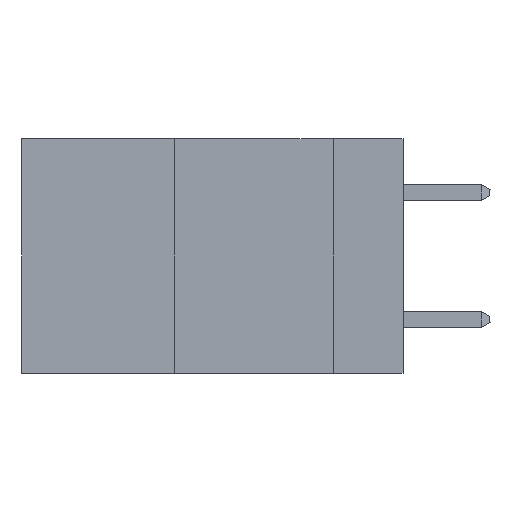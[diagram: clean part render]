
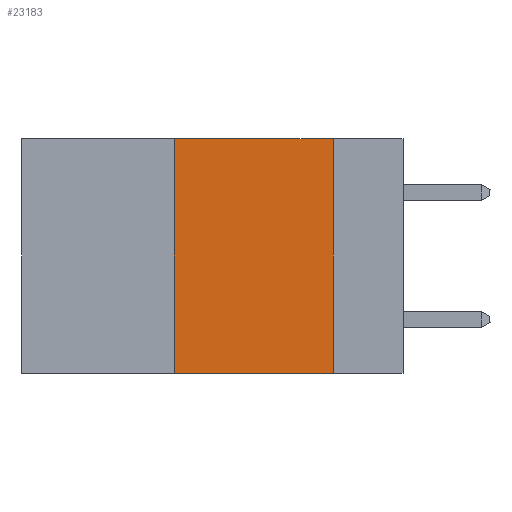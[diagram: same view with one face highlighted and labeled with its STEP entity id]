
A CAD part, left-side view. The second image highlights one B-rep face of the part: STEP entity #23183.
In plain terms, the highlighted planar face has unit normal (-1, 0, 0).
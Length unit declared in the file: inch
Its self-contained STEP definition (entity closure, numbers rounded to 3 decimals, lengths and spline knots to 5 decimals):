
#1402 = DIRECTION ( 'NONE',  ( 0., 0., -1. ) ) ;
#1811 = CARTESIAN_POINT ( 'NONE',  ( 0., 0.6, 0. ) ) ;
#2018 = EDGE_CURVE ( 'NONE', #37760, #12772, #20050, .T. ) ;
#2863 = EDGE_CURVE ( 'NONE', #10679, #37760, #13141, .T. ) ;
#3066 = VECTOR ( 'NONE', #6908, 39.37008 ) ;
#6908 = DIRECTION ( 'NONE',  ( 0., 0., 1. ) ) ;
#8728 = VECTOR ( 'NONE', #30118, 39.37008 ) ;
#8920 = EDGE_CURVE ( 'NONE', #46099, #10679, #19855, .T. ) ;
#9226 = CARTESIAN_POINT ( 'NONE',  ( 0., 0.36, -0.37 ) ) ;
#10679 = VERTEX_POINT ( 'NONE', #29574 ) ;
#11823 = AXIS2_PLACEMENT_3D ( 'NONE', #1811, #25742, #17429 ) ;
#12772 = VERTEX_POINT ( 'NONE', #44998 ) ;
#13032 = CARTESIAN_POINT ( 'NONE',  ( 0., 0.11, 0. ) ) ;
#13141 = LINE ( 'NONE', #18152, #8728 ) ;
#15585 = ORIENTED_EDGE ( 'NONE', *, *, #2018, .F. ) ;
#17429 = DIRECTION ( 'NONE',  ( 0., 0., -1. ) ) ;
#17936 = PLANE ( 'NONE',  #11823 ) ;
#18152 = CARTESIAN_POINT ( 'NONE',  ( 0., 0.6, 0. ) ) ;
#19242 = CARTESIAN_POINT ( 'NONE',  ( 0., 0.36, 0. ) ) ;
#19348 = EDGE_LOOP ( 'NONE', ( #15585, #40892, #36220, #49140 ) ) ;
#19855 = LINE ( 'NONE', #19242, #3066 ) ;
#20050 = LINE ( 'NONE', #25315, #39928 ) ;
#21603 = EDGE_CURVE ( 'NONE', #46099, #12772, #36631, .T. ) ;
#23014 = CARTESIAN_POINT ( 'NONE',  ( 0., 0.6, -0.37 ) ) ;
#23183 = ADVANCED_FACE ( 'NONE', ( #37629 ), #17936, .F. ) ;
#25315 = CARTESIAN_POINT ( 'NONE',  ( 0., 0.11, 0. ) ) ;
#25742 = DIRECTION ( 'NONE',  ( 1., 0., 0. ) ) ;
#29574 = CARTESIAN_POINT ( 'NONE',  ( 0., 0.36, 0. ) ) ;
#30118 = DIRECTION ( 'NONE',  ( 0., -1., 0. ) ) ;
#31193 = DIRECTION ( 'NONE',  ( 0., -1., 0. ) ) ;
#36220 = ORIENTED_EDGE ( 'NONE', *, *, #8920, .F. ) ;
#36631 = LINE ( 'NONE', #23014, #42222 ) ;
#37629 = FACE_OUTER_BOUND ( 'NONE', #19348, .T. ) ;
#37760 = VERTEX_POINT ( 'NONE', #13032 ) ;
#39928 = VECTOR ( 'NONE', #1402, 39.37008 ) ;
#40892 = ORIENTED_EDGE ( 'NONE', *, *, #2863, .F. ) ;
#42222 = VECTOR ( 'NONE', #31193, 39.37008 ) ;
#44998 = CARTESIAN_POINT ( 'NONE',  ( 0., 0.11, -0.37 ) ) ;
#46099 = VERTEX_POINT ( 'NONE', #9226 ) ;
#49140 = ORIENTED_EDGE ( 'NONE', *, *, #21603, .T. ) ;
